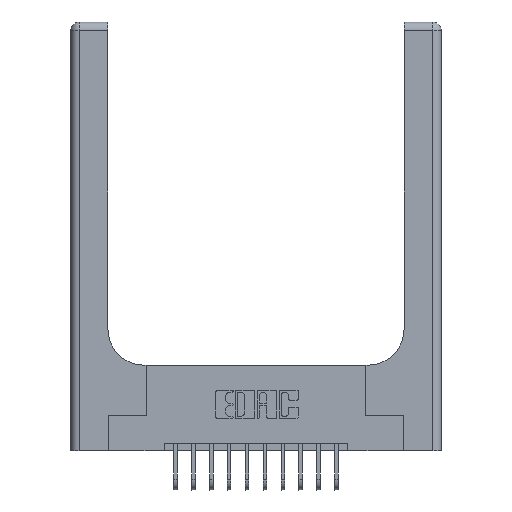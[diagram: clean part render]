
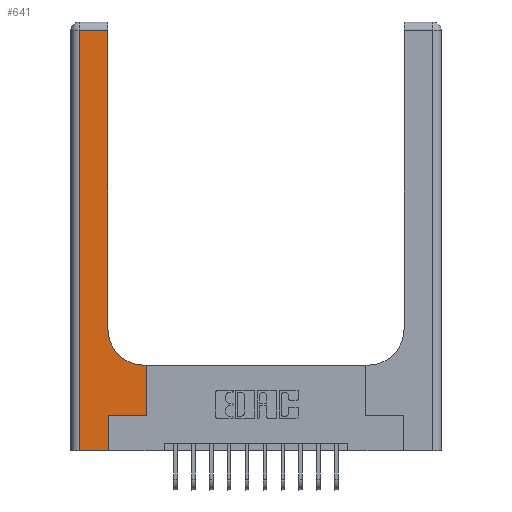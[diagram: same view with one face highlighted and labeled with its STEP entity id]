
A CAD part, top view. The second image highlights one B-rep face of the part: STEP entity #641.
In plain terms, the highlighted planar face has unit normal (0, 0, 1).
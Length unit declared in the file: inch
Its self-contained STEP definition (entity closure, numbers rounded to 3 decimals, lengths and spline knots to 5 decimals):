
#302 = VECTOR ( 'NONE', #6585, 39.37008 ) ;
#315 = DIRECTION ( 'NONE',  ( 1., 0., 0. ) ) ;
#410 = CARTESIAN_POINT ( 'NONE',  ( 0.51, 0.85, 0.37 ) ) ;
#418 = EDGE_CURVE ( 'NONE', #4920, #428, #15274, .T. ) ;
#428 = VERTEX_POINT ( 'NONE', #9380 ) ;
#641 = ADVANCED_FACE ( 'NONE', ( #10560 ), #10478, .F. ) ;
#1220 = VECTOR ( 'NONE', #8451, 39.37008 ) ;
#1285 = ORIENTED_EDGE ( 'NONE', *, *, #8419, .T. ) ;
#1698 = DIRECTION ( 'NONE',  ( 0., 0., -1. ) ) ;
#1939 = ORIENTED_EDGE ( 'NONE', *, *, #2591, .T. ) ;
#2272 = ORIENTED_EDGE ( 'NONE', *, *, #13356, .T. ) ;
#2591 = EDGE_CURVE ( 'NONE', #3757, #6559, #16327, .T. ) ;
#2838 = VECTOR ( 'NONE', #5100, 39.37008 ) ;
#2899 = LINE ( 'NONE', #16851, #1220 ) ;
#3145 = VERTEX_POINT ( 'NONE', #11929 ) ;
#3250 = ORIENTED_EDGE ( 'NONE', *, *, #13718, .T. ) ;
#3448 = LINE ( 'NONE', #11753, #8870 ) ;
#3757 = VERTEX_POINT ( 'NONE', #6122 ) ;
#4032 = CARTESIAN_POINT ( 'NONE',  ( 0., 2.94, 0.37 ) ) ;
#4194 = CARTESIAN_POINT ( 'NONE',  ( 0.528, 0.25, 0.37 ) ) ;
#4346 = EDGE_CURVE ( 'NONE', #6559, #4920, #13302, .T. ) ;
#4359 = VECTOR ( 'NONE', #12576, 39.37008 ) ;
#4748 = VERTEX_POINT ( 'NONE', #13468 ) ;
#4753 = CARTESIAN_POINT ( 'NONE',  ( 0.06, 3., 0.37 ) ) ;
#4920 = VERTEX_POINT ( 'NONE', #8741 ) ;
#5100 = DIRECTION ( 'NONE',  ( 0., 1., 0. ) ) ;
#5202 = CARTESIAN_POINT ( 'NONE',  ( 0.265, 0.25, 0.37 ) ) ;
#5542 = VERTEX_POINT ( 'NONE', #4194 ) ;
#5671 = VECTOR ( 'NONE', #13910, 39.37008 ) ;
#5773 = DIRECTION ( 'NONE',  ( 1., 0., 0. ) ) ;
#6122 = CARTESIAN_POINT ( 'NONE',  ( 0.51, 0.6, 0.37 ) ) ;
#6130 = DIRECTION ( 'NONE',  ( 0., 0., -1. ) ) ;
#6325 = CARTESIAN_POINT ( 'NONE',  ( 0., 3., 0.37 ) ) ;
#6394 = VECTOR ( 'NONE', #10837, 39.37008 ) ;
#6559 = VERTEX_POINT ( 'NONE', #13452 ) ;
#6585 = DIRECTION ( 'NONE',  ( 1., 0., 0. ) ) ;
#7102 = CARTESIAN_POINT ( 'NONE',  ( 0.528, 0.25, 0.37 ) ) ;
#7193 = ORIENTED_EDGE ( 'NONE', *, *, #14850, .T. ) ;
#7640 = EDGE_LOOP ( 'NONE', ( #12177, #17267, #1285, #2272, #13986, #3250, #16656, #7193, #1939 ) ) ;
#8365 = CARTESIAN_POINT ( 'NONE',  ( 0., 0., 0.37 ) ) ;
#8419 = EDGE_CURVE ( 'NONE', #428, #4748, #17405, .T. ) ;
#8451 = DIRECTION ( 'NONE',  ( 0., 1., 0. ) ) ;
#8741 = CARTESIAN_POINT ( 'NONE',  ( 0.26, 2.94, 0.37 ) ) ;
#8870 = VECTOR ( 'NONE', #16009, 39.37008 ) ;
#9000 = DIRECTION ( 'NONE',  ( -1., 0., 0. ) ) ;
#9380 = CARTESIAN_POINT ( 'NONE',  ( 0.06, 2.94, 0.37 ) ) ;
#10052 = CARTESIAN_POINT ( 'NONE',  ( 0.265, 0.25, 0.37 ) ) ;
#10306 = VECTOR ( 'NONE', #5773, 39.37008 ) ;
#10478 = PLANE ( 'NONE',  #13961 ) ;
#10560 = FACE_OUTER_BOUND ( 'NONE', #7640, .T. ) ;
#10837 = DIRECTION ( 'NONE',  ( 0., -1., 0. ) ) ;
#10883 = EDGE_CURVE ( 'NONE', #5542, #13132, #12391, .T. ) ;
#11753 = CARTESIAN_POINT ( 'NONE',  ( 0.26, 0.6, 0.37 ) ) ;
#11929 = CARTESIAN_POINT ( 'NONE',  ( 0.265, 0., 0.37 ) ) ;
#12177 = ORIENTED_EDGE ( 'NONE', *, *, #4346, .T. ) ;
#12391 = LINE ( 'NONE', #7102, #4359 ) ;
#12430 = VERTEX_POINT ( 'NONE', #10052 ) ;
#12576 = DIRECTION ( 'NONE',  ( 0., 1., 0. ) ) ;
#13132 = VERTEX_POINT ( 'NONE', #17938 ) ;
#13302 = LINE ( 'NONE', #13488, #2838 ) ;
#13356 = EDGE_CURVE ( 'NONE', #4748, #3145, #15352, .T. ) ;
#13452 = CARTESIAN_POINT ( 'NONE',  ( 0.26, 0.85, 0.37 ) ) ;
#13468 = CARTESIAN_POINT ( 'NONE',  ( 0.06, 0., 0.37 ) ) ;
#13488 = CARTESIAN_POINT ( 'NONE',  ( 0.26, 3., 0.37 ) ) ;
#13718 = EDGE_CURVE ( 'NONE', #12430, #5542, #13778, .T. ) ;
#13778 = LINE ( 'NONE', #5202, #302 ) ;
#13910 = DIRECTION ( 'NONE',  ( -1., 0., 0. ) ) ;
#13961 = AXIS2_PLACEMENT_3D ( 'NONE', #6325, #6130, #9000 ) ;
#13986 = ORIENTED_EDGE ( 'NONE', *, *, #14646, .T. ) ;
#14646 = EDGE_CURVE ( 'NONE', #3145, #12430, #2899, .T. ) ;
#14850 = EDGE_CURVE ( 'NONE', #13132, #3757, #3448, .T. ) ;
#15274 = LINE ( 'NONE', #4032, #5671 ) ;
#15352 = LINE ( 'NONE', #8365, #10306 ) ;
#16009 = DIRECTION ( 'NONE',  ( -1., 0., 0. ) ) ;
#16327 = CIRCLE ( 'NONE', #17814, 0.25 ) ;
#16656 = ORIENTED_EDGE ( 'NONE', *, *, #10883, .T. ) ;
#16851 = CARTESIAN_POINT ( 'NONE',  ( 0.265, 0., 0.37 ) ) ;
#17267 = ORIENTED_EDGE ( 'NONE', *, *, #418, .T. ) ;
#17405 = LINE ( 'NONE', #4753, #6394 ) ;
#17814 = AXIS2_PLACEMENT_3D ( 'NONE', #410, #1698, #315 ) ;
#17938 = CARTESIAN_POINT ( 'NONE',  ( 0.528, 0.6, 0.37 ) ) ;
